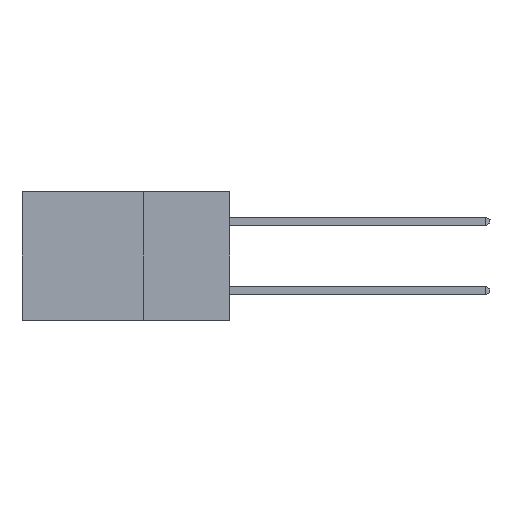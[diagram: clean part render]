
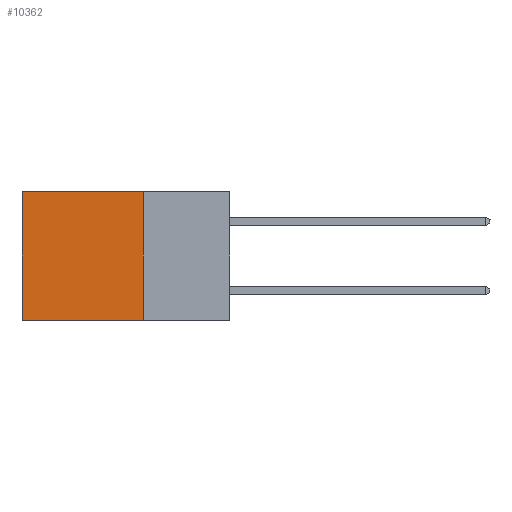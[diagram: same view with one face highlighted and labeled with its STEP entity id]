
A CAD part, left-side view. The second image highlights one B-rep face of the part: STEP entity #10362.
In plain terms, the highlighted planar face has unit normal (-1, 0, 0).
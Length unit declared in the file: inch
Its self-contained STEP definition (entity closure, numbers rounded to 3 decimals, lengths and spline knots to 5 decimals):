
#393 = DIRECTION ( 'NONE',  ( 0., 0., -1. ) ) ;
#730 = AXIS2_PLACEMENT_3D ( 'NONE', #9811, #6114, #11741 ) ;
#788 = EDGE_CURVE ( 'NONE', #13922, #4994, #4089, .T. ) ;
#1466 = CARTESIAN_POINT ( 'NONE',  ( 0.298, 0.6, -0.37 ) ) ;
#1805 = DIRECTION ( 'NONE',  ( 0., 1., 0. ) ) ;
#2482 = PLANE ( 'NONE',  #730 ) ;
#2538 = VECTOR ( 'NONE', #21292, 39.37008 ) ;
#2664 = EDGE_CURVE ( 'NONE', #22231, #7082, #4271, .T. ) ;
#2961 = CARTESIAN_POINT ( 'NONE',  ( 0.298, 0.25, 0. ) ) ;
#3513 = VECTOR ( 'NONE', #393, 39.37008 ) ;
#4089 = LINE ( 'NONE', #22098, #3513 ) ;
#4271 = LINE ( 'NONE', #2961, #2538 ) ;
#4994 = VERTEX_POINT ( 'NONE', #1466 ) ;
#6114 = DIRECTION ( 'NONE',  ( 1., 0., 0. ) ) ;
#7082 = VERTEX_POINT ( 'NONE', #12011 ) ;
#8480 = EDGE_CURVE ( 'NONE', #22231, #13922, #11404, .T. ) ;
#9811 = CARTESIAN_POINT ( 'NONE',  ( 0.298, 0.25, 0. ) ) ;
#10362 = ADVANCED_FACE ( 'NONE', ( #19251 ), #2482, .F. ) ;
#10856 = CARTESIAN_POINT ( 'NONE',  ( 0.298, 0.25, 0. ) ) ;
#11404 = LINE ( 'NONE', #10856, #11955 ) ;
#11520 = EDGE_LOOP ( 'NONE', ( #14267, #13884, #17587, #13820 ) ) ;
#11741 = DIRECTION ( 'NONE',  ( 0., 0., -1. ) ) ;
#11955 = VECTOR ( 'NONE', #18026, 39.37008 ) ;
#12011 = CARTESIAN_POINT ( 'NONE',  ( 0.298, 0.25, -0.37 ) ) ;
#13820 = ORIENTED_EDGE ( 'NONE', *, *, #8480, .T. ) ;
#13884 = ORIENTED_EDGE ( 'NONE', *, *, #19427, .F. ) ;
#13922 = VERTEX_POINT ( 'NONE', #20257 ) ;
#14267 = ORIENTED_EDGE ( 'NONE', *, *, #788, .T. ) ;
#17587 = ORIENTED_EDGE ( 'NONE', *, *, #2664, .F. ) ;
#18026 = DIRECTION ( 'NONE',  ( 0., 1., 0. ) ) ;
#19251 = FACE_OUTER_BOUND ( 'NONE', #11520, .T. ) ;
#19355 = CARTESIAN_POINT ( 'NONE',  ( 0.298, 0.25, 0. ) ) ;
#19427 = EDGE_CURVE ( 'NONE', #7082, #4994, #22169, .T. ) ;
#20186 = CARTESIAN_POINT ( 'NONE',  ( 0.298, 0.25, -0.37 ) ) ;
#20257 = CARTESIAN_POINT ( 'NONE',  ( 0.298, 0.6, 0. ) ) ;
#20470 = VECTOR ( 'NONE', #1805, 39.37008 ) ;
#21292 = DIRECTION ( 'NONE',  ( 0., 0., -1. ) ) ;
#22098 = CARTESIAN_POINT ( 'NONE',  ( 0.298, 0.6, 0. ) ) ;
#22169 = LINE ( 'NONE', #20186, #20470 ) ;
#22231 = VERTEX_POINT ( 'NONE', #19355 ) ;
